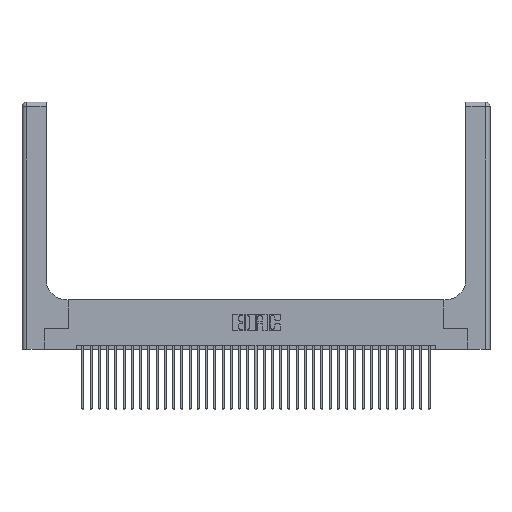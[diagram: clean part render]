
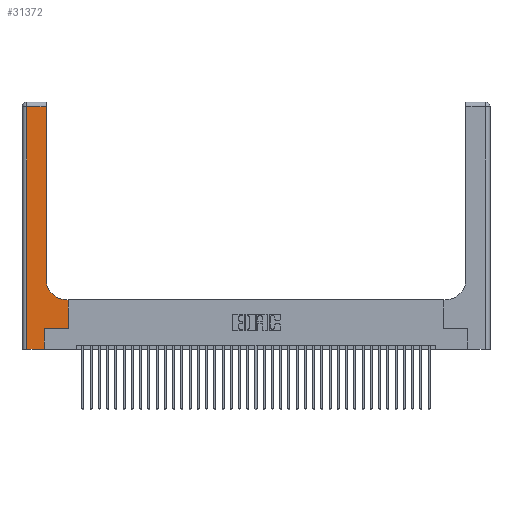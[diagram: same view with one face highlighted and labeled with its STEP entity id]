
A CAD part, top view. The second image highlights one B-rep face of the part: STEP entity #31372.
In plain terms, the highlighted planar face has unit normal (0, 0, 1).
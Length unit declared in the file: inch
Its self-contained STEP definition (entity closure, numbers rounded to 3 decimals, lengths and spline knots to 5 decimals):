
#3504 = EDGE_LOOP ( 'NONE', ( #28837, #23763, #32598, #26556, #28397, #5485, #21416, #38211, #9309 ) ) ;
#3509 = DIRECTION ( 'NONE',  ( 0., 0., -1. ) ) ;
#3513 = FACE_OUTER_BOUND ( 'NONE', #3504, .T. ) ;
#3537 = DIRECTION ( 'NONE',  ( -1., 0., 0. ) ) ;
#4415 = LINE ( 'NONE', #8129, #35324 ) ;
#5485 = ORIENTED_EDGE ( 'NONE', *, *, #19290, .T. ) ;
#5602 = VECTOR ( 'NONE', #28730, 39.37008 ) ;
#5634 = CARTESIAN_POINT ( 'NONE',  ( 0.269, 0., 0.37 ) ) ;
#5863 = AXIS2_PLACEMENT_3D ( 'NONE', #11789, #32655, #14826 ) ;
#6036 = DIRECTION ( 'NONE',  ( 0., -1., 0. ) ) ;
#6679 = AXIS2_PLACEMENT_3D ( 'NONE', #21512, #3509, #24513 ) ;
#7553 = DIRECTION ( 'NONE',  ( 1., 0., 0. ) ) ;
#7971 = EDGE_CURVE ( 'NONE', #10853, #12736, #21251, .T. ) ;
#8129 = CARTESIAN_POINT ( 'NONE',  ( 0., 2.94, 0.37 ) ) ;
#8146 = EDGE_CURVE ( 'NONE', #34853, #35449, #21696, .T. ) ;
#8233 = VECTOR ( 'NONE', #3537, 39.37008 ) ;
#8453 = DIRECTION ( 'NONE',  ( 1., 0., 0. ) ) ;
#9309 = ORIENTED_EDGE ( 'NONE', *, *, #14948, .T. ) ;
#10041 = EDGE_CURVE ( 'NONE', #25593, #24563, #16854, .T. ) ;
#10853 = VERTEX_POINT ( 'NONE', #11802 ) ;
#11724 = LINE ( 'NONE', #25775, #5602 ) ;
#11789 = CARTESIAN_POINT ( 'NONE',  ( 0.5415, 0.85, 0.37 ) ) ;
#11802 = CARTESIAN_POINT ( 'NONE',  ( 0.06, 0., 0.37 ) ) ;
#12070 = VERTEX_POINT ( 'NONE', #35485 ) ;
#12209 = CARTESIAN_POINT ( 'NONE',  ( 0.2915, 3., 0.37 ) ) ;
#12547 = CARTESIAN_POINT ( 'NONE',  ( 0.2915, 0.6, 0.37 ) ) ;
#12736 = VERTEX_POINT ( 'NONE', #5634 ) ;
#13316 = EDGE_CURVE ( 'NONE', #35449, #16736, #4415, .T. ) ;
#13635 = EDGE_CURVE ( 'NONE', #24563, #13747, #24110, .T. ) ;
#13747 = VERTEX_POINT ( 'NONE', #30495 ) ;
#14826 = DIRECTION ( 'NONE',  ( 1., 0., 0. ) ) ;
#14948 = EDGE_CURVE ( 'NONE', #13747, #34853, #32325, .T. ) ;
#15914 = VECTOR ( 'NONE', #21082, 39.37008 ) ;
#16616 = VECTOR ( 'NONE', #6036, 39.37008 ) ;
#16736 = VERTEX_POINT ( 'NONE', #21683 ) ;
#16854 = LINE ( 'NONE', #35956, #15914 ) ;
#19290 = EDGE_CURVE ( 'NONE', #12070, #25593, #24532, .T. ) ;
#20324 = VECTOR ( 'NONE', #8453, 39.37008 ) ;
#21082 = DIRECTION ( 'NONE',  ( 0., 1., 0. ) ) ;
#21251 = LINE ( 'NONE', #29284, #20324 ) ;
#21416 = ORIENTED_EDGE ( 'NONE', *, *, #10041, .T. ) ;
#21512 = CARTESIAN_POINT ( 'NONE',  ( 0., 3., 0.37 ) ) ;
#21683 = CARTESIAN_POINT ( 'NONE',  ( 0.06, 2.94, 0.37 ) ) ;
#21696 = LINE ( 'NONE', #12209, #31470 ) ;
#23137 = DIRECTION ( 'NONE',  ( -1., 0., 0. ) ) ;
#23487 = CARTESIAN_POINT ( 'NONE',  ( 0.5585, 0.6, 0.37 ) ) ;
#23763 = ORIENTED_EDGE ( 'NONE', *, *, #13316, .T. ) ;
#24110 = LINE ( 'NONE', #12547, #8233 ) ;
#24513 = DIRECTION ( 'NONE',  ( -1., 0., 0. ) ) ;
#24532 = LINE ( 'NONE', #25425, #26417 ) ;
#24553 = LINE ( 'NONE', #38816, #16616 ) ;
#24563 = VERTEX_POINT ( 'NONE', #23487 ) ;
#25425 = CARTESIAN_POINT ( 'NONE',  ( 0.269, 0.25, 0.37 ) ) ;
#25593 = VERTEX_POINT ( 'NONE', #28200 ) ;
#25775 = CARTESIAN_POINT ( 'NONE',  ( 0.269, 0., 0.37 ) ) ;
#26417 = VECTOR ( 'NONE', #7553, 39.37008 ) ;
#26556 = ORIENTED_EDGE ( 'NONE', *, *, #7971, .T. ) ;
#27381 = CARTESIAN_POINT ( 'NONE',  ( 0.2915, 2.94, 0.37 ) ) ;
#28200 = CARTESIAN_POINT ( 'NONE',  ( 0.5585, 0.25, 0.37 ) ) ;
#28397 = ORIENTED_EDGE ( 'NONE', *, *, #28747, .T. ) ;
#28730 = DIRECTION ( 'NONE',  ( 0., 1., 0. ) ) ;
#28747 = EDGE_CURVE ( 'NONE', #12736, #12070, #11724, .T. ) ;
#28837 = ORIENTED_EDGE ( 'NONE', *, *, #8146, .T. ) ;
#29284 = CARTESIAN_POINT ( 'NONE',  ( 0., 0., 0.37 ) ) ;
#30350 = PLANE ( 'NONE',  #6679 ) ;
#30495 = CARTESIAN_POINT ( 'NONE',  ( 0.5415, 0.6, 0.37 ) ) ;
#31372 = ADVANCED_FACE ( 'NONE', ( #3513 ), #30350, .F. ) ;
#31470 = VECTOR ( 'NONE', #33051, 39.37008 ) ;
#32325 = CIRCLE ( 'NONE', #5863, 0.25 ) ;
#32598 = ORIENTED_EDGE ( 'NONE', *, *, #35993, .T. ) ;
#32655 = DIRECTION ( 'NONE',  ( 0., 0., -1. ) ) ;
#33051 = DIRECTION ( 'NONE',  ( 0., 1., 0. ) ) ;
#33251 = CARTESIAN_POINT ( 'NONE',  ( 0.2915, 0.85, 0.37 ) ) ;
#34853 = VERTEX_POINT ( 'NONE', #33251 ) ;
#35324 = VECTOR ( 'NONE', #23137, 39.37008 ) ;
#35449 = VERTEX_POINT ( 'NONE', #27381 ) ;
#35485 = CARTESIAN_POINT ( 'NONE',  ( 0.269, 0.25, 0.37 ) ) ;
#35956 = CARTESIAN_POINT ( 'NONE',  ( 0.5585, 0.25, 0.37 ) ) ;
#35993 = EDGE_CURVE ( 'NONE', #16736, #10853, #24553, .T. ) ;
#38211 = ORIENTED_EDGE ( 'NONE', *, *, #13635, .T. ) ;
#38816 = CARTESIAN_POINT ( 'NONE',  ( 0.06, 3., 0.37 ) ) ;
